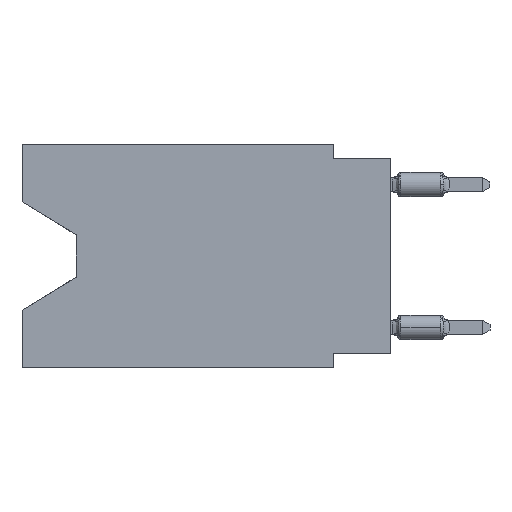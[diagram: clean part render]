
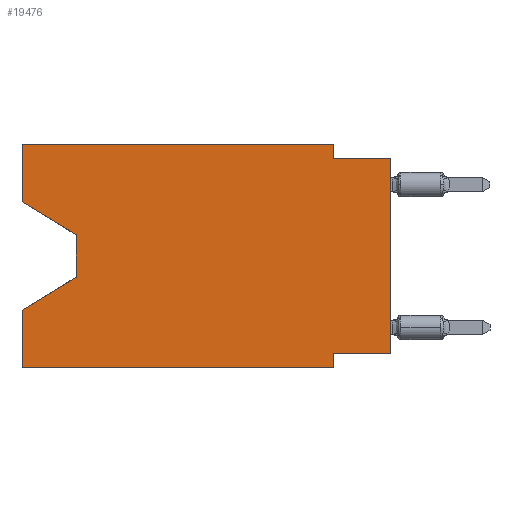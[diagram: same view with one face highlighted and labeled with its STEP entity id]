
A CAD part, left-side view. The second image highlights one B-rep face of the part: STEP entity #19476.
In plain terms, the highlighted planar face has unit normal (-1, 0, 0).
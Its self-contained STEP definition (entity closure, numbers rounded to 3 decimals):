
#149 = VERTEX_POINT ( 'NONE', #9179 ) ;
#156 = LINE ( 'NONE', #5915, #7962 ) ;
#289 = AXIS2_PLACEMENT_3D ( 'NONE', #4136, #2513, #801 ) ;
#554 = LINE ( 'NONE', #8140, #19135 ) ;
#563 = CARTESIAN_POINT ( 'NONE',  ( 0., 16.383, -2.546 ) ) ;
#801 = DIRECTION ( 'NONE',  ( 0., 0., -1. ) ) ;
#895 = PLANE ( 'NONE',  #289 ) ;
#939 = EDGE_CURVE ( 'NONE', #149, #11881, #14460, .T. ) ;
#1191 = CARTESIAN_POINT ( 'NONE',  ( 0., 13.97, -4.013 ) ) ;
#1393 = DIRECTION ( 'NONE',  ( 0., 0., -1. ) ) ;
#1467 = ORIENTED_EDGE ( 'NONE', *, *, #18647, .F. ) ;
#1720 = CARTESIAN_POINT ( 'NONE',  ( 0., 2.54, 0. ) ) ;
#1822 = CARTESIAN_POINT ( 'NONE',  ( 0., 2.54, -9.906 ) ) ;
#1873 = CARTESIAN_POINT ( 'NONE',  ( 0., 0., 0. ) ) ;
#2076 = VERTEX_POINT ( 'NONE', #19499 ) ;
#2136 = CARTESIAN_POINT ( 'NONE',  ( 0., 16.383, -2.546 ) ) ;
#2368 = LINE ( 'NONE', #14711, #8991 ) ;
#2513 = DIRECTION ( 'NONE',  ( 1., 0., 0. ) ) ;
#2965 = DIRECTION ( 'NONE',  ( 0., 0., -1. ) ) ;
#3441 = EDGE_CURVE ( 'NONE', #13139, #7631, #11931, .T. ) ;
#3735 = ORIENTED_EDGE ( 'NONE', *, *, #3441, .T. ) ;
#3791 = DIRECTION ( 'NONE',  ( 0., 1., 0. ) ) ;
#4136 = CARTESIAN_POINT ( 'NONE',  ( 0., 16.383, 0. ) ) ;
#4378 = EDGE_CURVE ( 'NONE', #17679, #8552, #156, .T. ) ;
#5063 = CARTESIAN_POINT ( 'NONE',  ( 0., 13.97, -5.893 ) ) ;
#5157 = VECTOR ( 'NONE', #10166, 1000. ) ;
#5327 = VECTOR ( 'NONE', #11329, 1000. ) ;
#5730 = FACE_OUTER_BOUND ( 'NONE', #7171, .T. ) ;
#5915 = CARTESIAN_POINT ( 'NONE',  ( 0., 16.383, 0. ) ) ;
#6131 = EDGE_CURVE ( 'NONE', #17965, #7316, #14198, .T. ) ;
#6326 = LINE ( 'NONE', #1873, #7984 ) ;
#6387 = VERTEX_POINT ( 'NONE', #13874 ) ;
#6512 = VERTEX_POINT ( 'NONE', #2136 ) ;
#6614 = DIRECTION ( 'NONE',  ( 0., 0., 1. ) ) ;
#7171 = EDGE_LOOP ( 'NONE', ( #12346, #3735, #16691, #14918, #18302, #1467, #15953, #11809, #13447, #8666, #15713, #13811 ) ) ;
#7222 = VERTEX_POINT ( 'NONE', #9075 ) ;
#7267 = CARTESIAN_POINT ( 'NONE',  ( 0., 13.97, -4.013 ) ) ;
#7316 = VERTEX_POINT ( 'NONE', #13099 ) ;
#7379 = DIRECTION ( 'NONE',  ( 0., 0.855, -0.519 ) ) ;
#7631 = VERTEX_POINT ( 'NONE', #5063 ) ;
#7775 = CARTESIAN_POINT ( 'NONE',  ( 0., 13.97, -5.893 ) ) ;
#7962 = VECTOR ( 'NONE', #10981, 1000. ) ;
#7984 = VECTOR ( 'NONE', #17368, 1000. ) ;
#8140 = CARTESIAN_POINT ( 'NONE',  ( 0., 16.383, 0. ) ) ;
#8231 = CARTESIAN_POINT ( 'NONE',  ( 0., 0., -9.271 ) ) ;
#8487 = CARTESIAN_POINT ( 'NONE',  ( 0., 2.54, 0. ) ) ;
#8552 = VERTEX_POINT ( 'NONE', #8487 ) ;
#8666 = ORIENTED_EDGE ( 'NONE', *, *, #17646, .F. ) ;
#8991 = VECTOR ( 'NONE', #11378, 1000. ) ;
#9075 = CARTESIAN_POINT ( 'NONE',  ( 0., 2.54, -0.635 ) ) ;
#9132 = DIRECTION ( 'NONE',  ( 0., -1., 0. ) ) ;
#9179 = CARTESIAN_POINT ( 'NONE',  ( 0., 16.383, -9.906 ) ) ;
#9711 = VECTOR ( 'NONE', #9886, 1000. ) ;
#9886 = DIRECTION ( 'NONE',  ( 0., -0.855, -0.519 ) ) ;
#10166 = DIRECTION ( 'NONE',  ( 0., 0., 1. ) ) ;
#10672 = EDGE_CURVE ( 'NONE', #6512, #17679, #16253, .T. ) ;
#10841 = LINE ( 'NONE', #1720, #10894 ) ;
#10894 = VECTOR ( 'NONE', #2965, 1000. ) ;
#10981 = DIRECTION ( 'NONE',  ( 0., -1., 0. ) ) ;
#11329 = DIRECTION ( 'NONE',  ( 0., -1., 0. ) ) ;
#11378 = DIRECTION ( 'NONE',  ( 0., 0., -1. ) ) ;
#11781 = EDGE_CURVE ( 'NONE', #149, #2076, #554, .T. ) ;
#11809 = ORIENTED_EDGE ( 'NONE', *, *, #18034, .T. ) ;
#11881 = VERTEX_POINT ( 'NONE', #1822 ) ;
#11931 = LINE ( 'NONE', #7267, #19927 ) ;
#12263 = LINE ( 'NONE', #12369, #13994 ) ;
#12346 = ORIENTED_EDGE ( 'NONE', *, *, #17027, .T. ) ;
#12359 = EDGE_CURVE ( 'NONE', #7222, #6387, #12263, .T. ) ;
#12369 = CARTESIAN_POINT ( 'NONE',  ( 0., 0., -0.635 ) ) ;
#12503 = CARTESIAN_POINT ( 'NONE',  ( 0., 0., -9.271 ) ) ;
#13099 = CARTESIAN_POINT ( 'NONE',  ( 0., 2.54, -9.271 ) ) ;
#13139 = VERTEX_POINT ( 'NONE', #1191 ) ;
#13447 = ORIENTED_EDGE ( 'NONE', *, *, #12359, .F. ) ;
#13811 = ORIENTED_EDGE ( 'NONE', *, *, #10672, .F. ) ;
#13874 = CARTESIAN_POINT ( 'NONE',  ( 0., 0., -0.635 ) ) ;
#13994 = VECTOR ( 'NONE', #9132, 1000. ) ;
#14198 = LINE ( 'NONE', #8231, #15981 ) ;
#14427 = LINE ( 'NONE', #563, #9711 ) ;
#14460 = LINE ( 'NONE', #18994, #5327 ) ;
#14711 = CARTESIAN_POINT ( 'NONE',  ( 0., 2.54, -9.906 ) ) ;
#14918 = ORIENTED_EDGE ( 'NONE', *, *, #11781, .F. ) ;
#15713 = ORIENTED_EDGE ( 'NONE', *, *, #4378, .F. ) ;
#15953 = ORIENTED_EDGE ( 'NONE', *, *, #6131, .F. ) ;
#15981 = VECTOR ( 'NONE', #3791, 1000. ) ;
#16163 = VECTOR ( 'NONE', #7379, 1000. ) ;
#16253 = LINE ( 'NONE', #19453, #5157 ) ;
#16691 = ORIENTED_EDGE ( 'NONE', *, *, #19726, .T. ) ;
#16800 = LINE ( 'NONE', #7775, #16163 ) ;
#17014 = CARTESIAN_POINT ( 'NONE',  ( 0., 16.383, 0. ) ) ;
#17027 = EDGE_CURVE ( 'NONE', #6512, #13139, #14427, .T. ) ;
#17368 = DIRECTION ( 'NONE',  ( 0., 0., 1. ) ) ;
#17646 = EDGE_CURVE ( 'NONE', #8552, #7222, #10841, .T. ) ;
#17679 = VERTEX_POINT ( 'NONE', #17014 ) ;
#17965 = VERTEX_POINT ( 'NONE', #12503 ) ;
#18034 = EDGE_CURVE ( 'NONE', #17965, #6387, #6326, .T. ) ;
#18302 = ORIENTED_EDGE ( 'NONE', *, *, #939, .T. ) ;
#18647 = EDGE_CURVE ( 'NONE', #7316, #11881, #2368, .T. ) ;
#18994 = CARTESIAN_POINT ( 'NONE',  ( 0., 16.383, -9.906 ) ) ;
#19135 = VECTOR ( 'NONE', #6614, 1000. ) ;
#19453 = CARTESIAN_POINT ( 'NONE',  ( 0., 16.383, 0. ) ) ;
#19476 = ADVANCED_FACE ( 'NONE', ( #5730 ), #895, .F. ) ;
#19499 = CARTESIAN_POINT ( 'NONE',  ( 0., 16.383, -7.36 ) ) ;
#19726 = EDGE_CURVE ( 'NONE', #7631, #2076, #16800, .T. ) ;
#19927 = VECTOR ( 'NONE', #1393, 1000. ) ;
